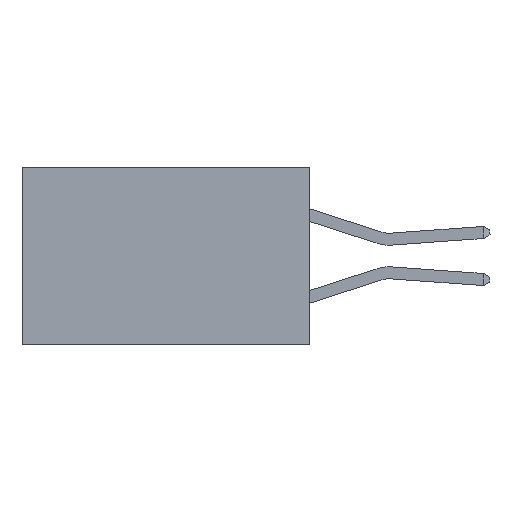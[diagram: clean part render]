
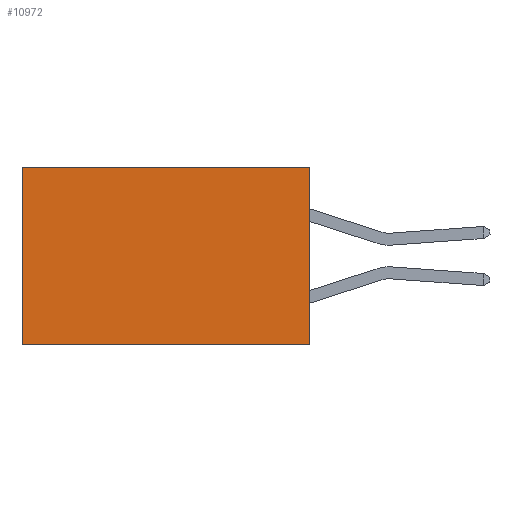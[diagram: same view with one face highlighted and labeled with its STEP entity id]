
A CAD part, left-side view. The second image highlights one B-rep face of the part: STEP entity #10972.
In plain terms, the highlighted planar face has unit normal (-1, 0, 0).
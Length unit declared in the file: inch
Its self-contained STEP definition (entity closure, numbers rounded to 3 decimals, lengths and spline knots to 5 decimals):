
#556 = VERTEX_POINT ( 'NONE', #18965 ) ;
#682 = EDGE_LOOP ( 'NONE', ( #5871, #5870, #11710, #14765 ) ) ;
#1538 = LINE ( 'NONE', #18216, #5482 ) ;
#2410 = CARTESIAN_POINT ( 'NONE',  ( 0.298, 0.6, 0. ) ) ;
#2896 = DIRECTION ( 'NONE',  ( 0., 1., 0. ) ) ;
#4614 = CARTESIAN_POINT ( 'NONE',  ( 0.298, 0., 0. ) ) ;
#5482 = VECTOR ( 'NONE', #14970, 39.37008 ) ;
#5870 = ORIENTED_EDGE ( 'NONE', *, *, #9818, .F. ) ;
#5871 = ORIENTED_EDGE ( 'NONE', *, *, #10950, .T. ) ;
#6528 = EDGE_CURVE ( 'NONE', #11775, #22487, #20558, .T. ) ;
#7396 = EDGE_CURVE ( 'NONE', #11775, #556, #15652, .T. ) ;
#9818 = EDGE_CURVE ( 'NONE', #556, #15135, #20085, .T. ) ;
#9859 = VECTOR ( 'NONE', #2896, 39.37008 ) ;
#10747 = CARTESIAN_POINT ( 'NONE',  ( 0.298, 0., 0. ) ) ;
#10950 = EDGE_CURVE ( 'NONE', #22487, #15135, #1538, .T. ) ;
#10972 = ADVANCED_FACE ( 'NONE', ( #15595 ), #20752, .F. ) ;
#11024 = DIRECTION ( 'NONE',  ( 0., 0., -1. ) ) ;
#11710 = ORIENTED_EDGE ( 'NONE', *, *, #7396, .F. ) ;
#11775 = VERTEX_POINT ( 'NONE', #19478 ) ;
#14765 = ORIENTED_EDGE ( 'NONE', *, *, #6528, .T. ) ;
#14970 = DIRECTION ( 'NONE',  ( 0., 0., -1. ) ) ;
#15135 = VERTEX_POINT ( 'NONE', #24770 ) ;
#15526 = VECTOR ( 'NONE', #20153, 39.37008 ) ;
#15595 = FACE_OUTER_BOUND ( 'NONE', #682, .T. ) ;
#15652 = LINE ( 'NONE', #18273, #18111 ) ;
#16112 = AXIS2_PLACEMENT_3D ( 'NONE', #10747, #24669, #11024 ) ;
#18111 = VECTOR ( 'NONE', #24563, 39.37008 ) ;
#18216 = CARTESIAN_POINT ( 'NONE',  ( 0.298, 0.6, 0. ) ) ;
#18273 = CARTESIAN_POINT ( 'NONE',  ( 0.298, 0., 0. ) ) ;
#18295 = CARTESIAN_POINT ( 'NONE',  ( 0.298, 0., -0.37 ) ) ;
#18965 = CARTESIAN_POINT ( 'NONE',  ( 0.298, 0., -0.37 ) ) ;
#19478 = CARTESIAN_POINT ( 'NONE',  ( 0.298, 0., 0. ) ) ;
#20085 = LINE ( 'NONE', #18295, #15526 ) ;
#20153 = DIRECTION ( 'NONE',  ( 0., 1., 0. ) ) ;
#20558 = LINE ( 'NONE', #4614, #9859 ) ;
#20752 = PLANE ( 'NONE',  #16112 ) ;
#22487 = VERTEX_POINT ( 'NONE', #2410 ) ;
#24563 = DIRECTION ( 'NONE',  ( 0., 0., -1. ) ) ;
#24669 = DIRECTION ( 'NONE',  ( 1., 0., 0. ) ) ;
#24770 = CARTESIAN_POINT ( 'NONE',  ( 0.298, 0.6, -0.37 ) ) ;
